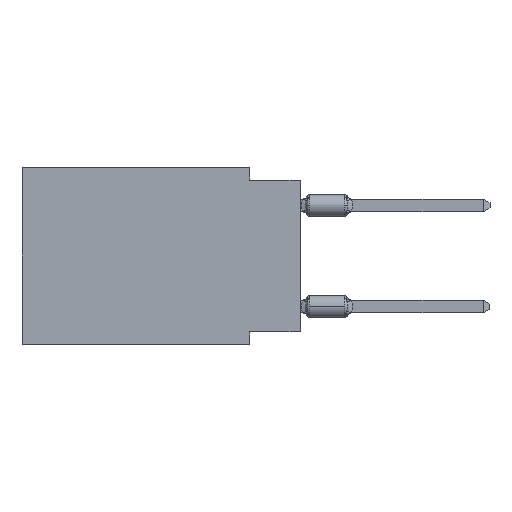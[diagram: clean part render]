
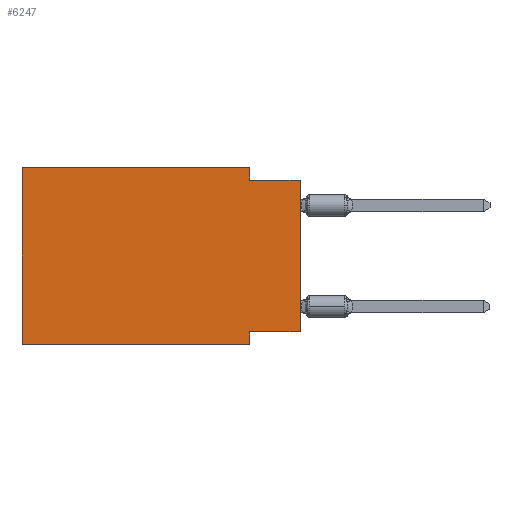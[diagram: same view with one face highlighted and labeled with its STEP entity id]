
A CAD part, left-side view. The second image highlights one B-rep face of the part: STEP entity #6247.
In plain terms, the highlighted planar face has unit normal (-1, 0, 0).
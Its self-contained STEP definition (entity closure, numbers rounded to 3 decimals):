
#5 = EDGE_CURVE ( 'NONE', #14459, #7431, #8785, .T. ) ;
#1343 = LINE ( 'NONE', #6681, #13335 ) ;
#1727 = DIRECTION ( 'NONE',  ( 0., 0., -1. ) ) ;
#2206 = LINE ( 'NONE', #5141, #3015 ) ;
#2617 = VECTOR ( 'NONE', #3706, 1000. ) ;
#2855 = DIRECTION ( 'NONE',  ( 0., 0., -1. ) ) ;
#2919 = CARTESIAN_POINT ( 'NONE',  ( 0., 13.97, -8.89 ) ) ;
#2980 = EDGE_CURVE ( 'NONE', #10777, #7656, #1343, .T. ) ;
#3015 = VECTOR ( 'NONE', #9462, 1000. ) ;
#3335 = VERTEX_POINT ( 'NONE', #7844 ) ;
#3706 = DIRECTION ( 'NONE',  ( 0., -1., 0. ) ) ;
#4465 = PLANE ( 'NONE',  #4853 ) ;
#4853 = AXIS2_PLACEMENT_3D ( 'NONE', #15627, #15451, #1727 ) ;
#5084 = LINE ( 'NONE', #10598, #2617 ) ;
#5141 = CARTESIAN_POINT ( 'NONE',  ( 0., 13.97, 0. ) ) ;
#5186 = EDGE_CURVE ( 'NONE', #7656, #7431, #14200, .T. ) ;
#5659 = EDGE_CURVE ( 'NONE', #8401, #7405, #13504, .T. ) ;
#5705 = VECTOR ( 'NONE', #14088, 1000. ) ;
#6247 = ADVANCED_FACE ( 'NONE', ( #14918 ), #4465, .F. ) ;
#6681 = CARTESIAN_POINT ( 'NONE',  ( 0., 0., -8.255 ) ) ;
#6881 = CARTESIAN_POINT ( 'NONE',  ( 0., 2.54, -8.89 ) ) ;
#7175 = CARTESIAN_POINT ( 'NONE',  ( 0., 2.54, -8.89 ) ) ;
#7405 = VERTEX_POINT ( 'NONE', #18030 ) ;
#7431 = VERTEX_POINT ( 'NONE', #6881 ) ;
#7643 = DIRECTION ( 'NONE',  ( 0., 0., 1. ) ) ;
#7656 = VERTEX_POINT ( 'NONE', #7771 ) ;
#7771 = CARTESIAN_POINT ( 'NONE',  ( 0., 2.54, -8.255 ) ) ;
#7844 = CARTESIAN_POINT ( 'NONE',  ( 0., 13.97, 0. ) ) ;
#8401 = VERTEX_POINT ( 'NONE', #15682 ) ;
#8785 = LINE ( 'NONE', #2919, #5705 ) ;
#9462 = DIRECTION ( 'NONE',  ( 0., -1., 0. ) ) ;
#9468 = ORIENTED_EDGE ( 'NONE', *, *, #5659, .F. ) ;
#9695 = CARTESIAN_POINT ( 'NONE',  ( 0., 0., -0.635 ) ) ;
#9767 = LINE ( 'NONE', #12245, #10333 ) ;
#9955 = ORIENTED_EDGE ( 'NONE', *, *, #17841, .T. ) ;
#10007 = VERTEX_POINT ( 'NONE', #9695 ) ;
#10333 = VECTOR ( 'NONE', #16628, 1000. ) ;
#10405 = CARTESIAN_POINT ( 'NONE',  ( 0., 2.54, 0. ) ) ;
#10542 = ORIENTED_EDGE ( 'NONE', *, *, #2980, .F. ) ;
#10598 = CARTESIAN_POINT ( 'NONE',  ( 0., 0., -0.635 ) ) ;
#10610 = EDGE_CURVE ( 'NONE', #14459, #3335, #14486, .T. ) ;
#10639 = ORIENTED_EDGE ( 'NONE', *, *, #10610, .F. ) ;
#10777 = VERTEX_POINT ( 'NONE', #14091 ) ;
#11420 = EDGE_CURVE ( 'NONE', #7405, #10007, #5084, .T. ) ;
#12245 = CARTESIAN_POINT ( 'NONE',  ( 0., 0., 0. ) ) ;
#13114 = EDGE_LOOP ( 'NONE', ( #9955, #16705, #9468, #15578, #10639, #16049, #16207, #10542 ) ) ;
#13204 = CARTESIAN_POINT ( 'NONE',  ( 0., 13.97, 0. ) ) ;
#13335 = VECTOR ( 'NONE', #13790, 1000. ) ;
#13504 = LINE ( 'NONE', #10405, #17754 ) ;
#13790 = DIRECTION ( 'NONE',  ( 0., 1., 0. ) ) ;
#14088 = DIRECTION ( 'NONE',  ( 0., -1., 0. ) ) ;
#14091 = CARTESIAN_POINT ( 'NONE',  ( 0., 0., -8.255 ) ) ;
#14200 = LINE ( 'NONE', #7175, #14228 ) ;
#14228 = VECTOR ( 'NONE', #2855, 1000. ) ;
#14304 = CARTESIAN_POINT ( 'NONE',  ( 0., 13.97, -8.89 ) ) ;
#14459 = VERTEX_POINT ( 'NONE', #14304 ) ;
#14486 = LINE ( 'NONE', #13204, #16366 ) ;
#14612 = DIRECTION ( 'NONE',  ( 0., 0., -1. ) ) ;
#14918 = FACE_OUTER_BOUND ( 'NONE', #13114, .T. ) ;
#15451 = DIRECTION ( 'NONE',  ( 1., 0., 0. ) ) ;
#15578 = ORIENTED_EDGE ( 'NONE', *, *, #18088, .F. ) ;
#15627 = CARTESIAN_POINT ( 'NONE',  ( 0., 13.97, 0. ) ) ;
#15682 = CARTESIAN_POINT ( 'NONE',  ( 0., 2.54, 0. ) ) ;
#16049 = ORIENTED_EDGE ( 'NONE', *, *, #5, .T. ) ;
#16207 = ORIENTED_EDGE ( 'NONE', *, *, #5186, .F. ) ;
#16366 = VECTOR ( 'NONE', #7643, 1000. ) ;
#16628 = DIRECTION ( 'NONE',  ( 0., 0., 1. ) ) ;
#16705 = ORIENTED_EDGE ( 'NONE', *, *, #11420, .F. ) ;
#17754 = VECTOR ( 'NONE', #14612, 1000. ) ;
#17841 = EDGE_CURVE ( 'NONE', #10777, #10007, #9767, .T. ) ;
#18030 = CARTESIAN_POINT ( 'NONE',  ( 0., 2.54, -0.635 ) ) ;
#18088 = EDGE_CURVE ( 'NONE', #3335, #8401, #2206, .T. ) ;
